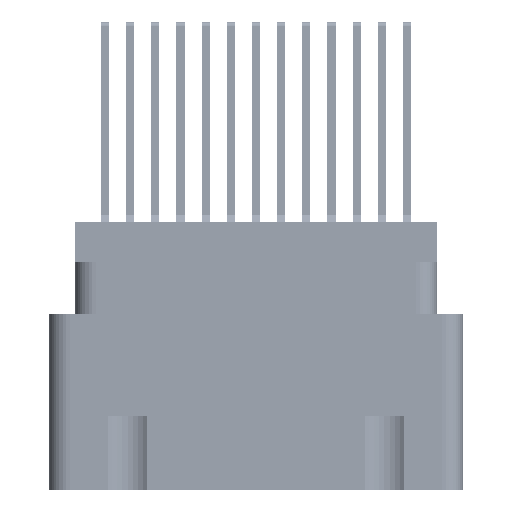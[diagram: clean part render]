
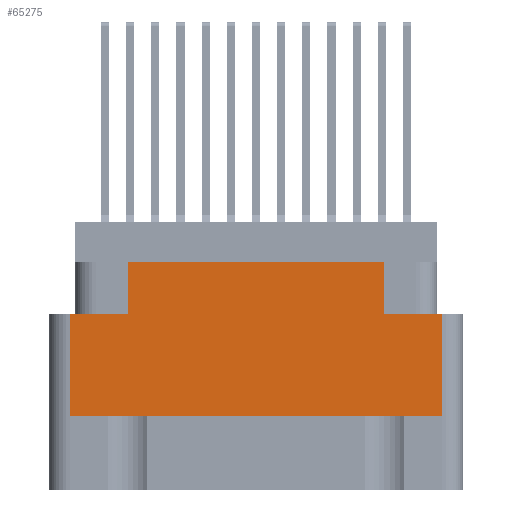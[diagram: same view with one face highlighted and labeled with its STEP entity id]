
A CAD part, left-side view. The second image highlights one B-rep face of the part: STEP entity #65275.
In plain terms, the highlighted planar face has unit normal (-1, 0, 0).
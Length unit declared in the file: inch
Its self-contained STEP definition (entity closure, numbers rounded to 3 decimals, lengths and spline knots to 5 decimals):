
#443 = EDGE_CURVE ( 'NONE', #9900, #51741, #32669, .T. ) ;
#1588 = EDGE_CURVE ( 'NONE', #57673, #62723, #53840, .T. ) ;
#2402 = VECTOR ( 'NONE', #6913, 39.37008 ) ;
#3005 = LINE ( 'NONE', #14404, #36652 ) ;
#4702 = VERTEX_POINT ( 'NONE', #46998 ) ;
#6913 = DIRECTION ( 'NONE',  ( 0., -1., 0. ) ) ;
#7117 = EDGE_CURVE ( 'NONE', #44417, #58917, #3005, .T. ) ;
#7972 = VECTOR ( 'NONE', #56697, 39.37008 ) ;
#8158 = VECTOR ( 'NONE', #14622, 39.37008 ) ;
#8340 = DIRECTION ( 'NONE',  ( 0., 0., 1. ) ) ;
#8395 = CARTESIAN_POINT ( 'NONE',  ( -1.359, 0.3825, -0.274 ) ) ;
#9900 = VERTEX_POINT ( 'NONE', #47970 ) ;
#10127 = LINE ( 'NONE', #64740, #15343 ) ;
#12887 = DIRECTION ( 'NONE',  ( 0., 0., 1. ) ) ;
#14404 = CARTESIAN_POINT ( 'NONE',  ( -1.359, -0.3825, -0.274 ) ) ;
#14622 = DIRECTION ( 'NONE',  ( 0., 0., 1. ) ) ;
#15086 = ORIENTED_EDGE ( 'NONE', *, *, #48684, .F. ) ;
#15343 = VECTOR ( 'NONE', #42792, 39.37008 ) ;
#15560 = CARTESIAN_POINT ( 'NONE',  ( -1.359, 0.617, -0.117 ) ) ;
#16257 = CARTESIAN_POINT ( 'NONE',  ( -1.359, -0.3825, -0.117 ) ) ;
#17685 = DIRECTION ( 'NONE',  ( 0., -1., 0. ) ) ;
#18436 = LINE ( 'NONE', #18844, #7972 ) ;
#18844 = CARTESIAN_POINT ( 'NONE',  ( -1.359, 0.555, -0.798 ) ) ;
#18960 = EDGE_CURVE ( 'NONE', #9900, #70760, #18436, .T. ) ;
#19439 = VECTOR ( 'NONE', #17685, 39.37008 ) ;
#20291 = LINE ( 'NONE', #15560, #19439 ) ;
#23623 = VECTOR ( 'NONE', #60475, 39.37008 ) ;
#25709 = EDGE_CURVE ( 'NONE', #70760, #57673, #10127, .T. ) ;
#26445 = CARTESIAN_POINT ( 'NONE',  ( -1.359, 0.3825, -0.274 ) ) ;
#27184 = CARTESIAN_POINT ( 'NONE',  ( -1.359, -0.555, -0.798 ) ) ;
#27941 = VECTOR ( 'NONE', #34043, 39.37008 ) ;
#32669 = LINE ( 'NONE', #45055, #2402 ) ;
#34043 = DIRECTION ( 'NONE',  ( 0., -1., 0. ) ) ;
#36652 = VECTOR ( 'NONE', #8340, 39.37008 ) ;
#42792 = DIRECTION ( 'NONE',  ( 0., -1., 0. ) ) ;
#43659 = AXIS2_PLACEMENT_3D ( 'NONE', #51212, #45917, #12887 ) ;
#44417 = VERTEX_POINT ( 'NONE', #69493 ) ;
#45055 = CARTESIAN_POINT ( 'NONE',  ( -1.359, 0., -0.274 ) ) ;
#45275 = LINE ( 'NONE', #26445, #8158 ) ;
#45917 = DIRECTION ( 'NONE',  ( -1., 0., 0. ) ) ;
#46998 = CARTESIAN_POINT ( 'NONE',  ( -1.359, 0.3825, -0.117 ) ) ;
#47970 = CARTESIAN_POINT ( 'NONE',  ( -1.359, 0.555, -0.274 ) ) ;
#48078 = ORIENTED_EDGE ( 'NONE', *, *, #18960, .T. ) ;
#48251 = EDGE_LOOP ( 'NONE', ( #67398, #48078, #50570, #51961, #57087, #60794, #48700, #15086 ) ) ;
#48684 = EDGE_CURVE ( 'NONE', #51741, #4702, #45275, .T. ) ;
#48700 = ORIENTED_EDGE ( 'NONE', *, *, #48722, .F. ) ;
#48722 = EDGE_CURVE ( 'NONE', #4702, #58917, #20291, .T. ) ;
#50570 = ORIENTED_EDGE ( 'NONE', *, *, #25709, .T. ) ;
#51212 = CARTESIAN_POINT ( 'NONE',  ( -1.359, -0.617, -0.798 ) ) ;
#51741 = VERTEX_POINT ( 'NONE', #8395 ) ;
#51961 = ORIENTED_EDGE ( 'NONE', *, *, #1588, .T. ) ;
#53840 = LINE ( 'NONE', #27184, #23623 ) ;
#54849 = CARTESIAN_POINT ( 'NONE',  ( -1.359, -0.555, -0.578 ) ) ;
#56535 = CARTESIAN_POINT ( 'NONE',  ( -1.359, 0., -0.274 ) ) ;
#56697 = DIRECTION ( 'NONE',  ( 0., 0., -1. ) ) ;
#57087 = ORIENTED_EDGE ( 'NONE', *, *, #61211, .F. ) ;
#57673 = VERTEX_POINT ( 'NONE', #54849 ) ;
#58619 = CARTESIAN_POINT ( 'NONE',  ( -1.359, 0.555, -0.578 ) ) ;
#58917 = VERTEX_POINT ( 'NONE', #16257 ) ;
#60475 = DIRECTION ( 'NONE',  ( 0., 0., 1. ) ) ;
#60794 = ORIENTED_EDGE ( 'NONE', *, *, #7117, .T. ) ;
#60930 = CARTESIAN_POINT ( 'NONE',  ( -1.359, -0.555, -0.274 ) ) ;
#61211 = EDGE_CURVE ( 'NONE', #44417, #62723, #65025, .T. ) ;
#62723 = VERTEX_POINT ( 'NONE', #60930 ) ;
#64740 = CARTESIAN_POINT ( 'NONE',  ( -1.359, 0., -0.578 ) ) ;
#65025 = LINE ( 'NONE', #56535, #27941 ) ;
#65275 = ADVANCED_FACE ( 'NONE', ( #65559 ), #67404, .T. ) ;
#65559 = FACE_OUTER_BOUND ( 'NONE', #48251, .T. ) ;
#67398 = ORIENTED_EDGE ( 'NONE', *, *, #443, .F. ) ;
#67404 = PLANE ( 'NONE',  #43659 ) ;
#69493 = CARTESIAN_POINT ( 'NONE',  ( -1.359, -0.3825, -0.274 ) ) ;
#70760 = VERTEX_POINT ( 'NONE', #58619 ) ;
